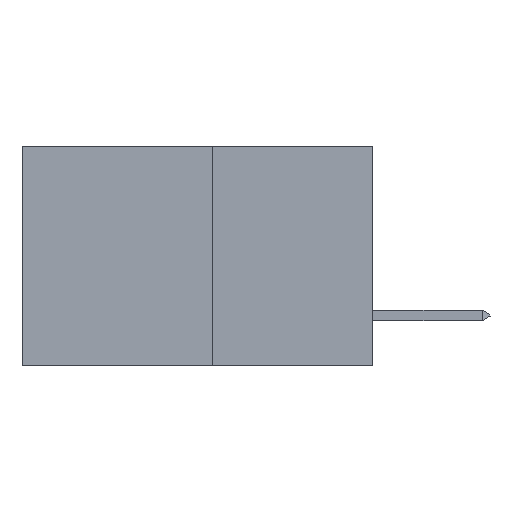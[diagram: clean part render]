
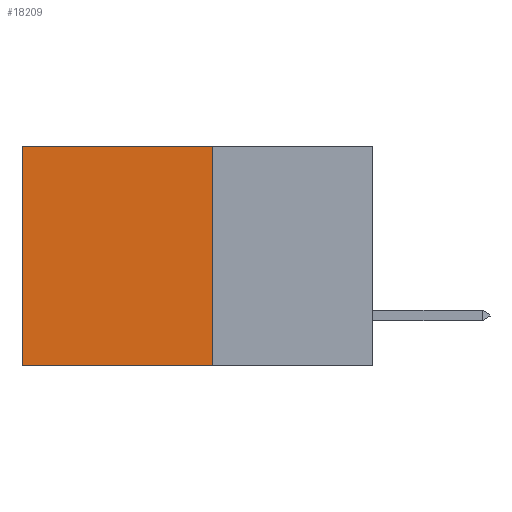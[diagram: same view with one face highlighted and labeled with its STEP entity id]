
A CAD part, left-side view. The second image highlights one B-rep face of the part: STEP entity #18209.
In plain terms, the highlighted planar face has unit normal (-1, 0, 0).
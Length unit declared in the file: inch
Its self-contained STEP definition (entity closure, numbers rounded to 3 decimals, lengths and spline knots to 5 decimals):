
#108 = EDGE_CURVE ( 'NONE', #5743, #16126, #417, .T. ) ;
#314 = DIRECTION ( 'NONE',  ( 0., 1., 0. ) ) ;
#417 = LINE ( 'NONE', #13929, #11786 ) ;
#859 = EDGE_CURVE ( 'NONE', #16126, #6185, #3263, .T. ) ;
#3263 = LINE ( 'NONE', #13642, #17883 ) ;
#4780 = EDGE_CURVE ( 'NONE', #5743, #17877, #18386, .T. ) ;
#4881 = DIRECTION ( 'NONE',  ( 0., 0., -1. ) ) ;
#4972 = EDGE_CURVE ( 'NONE', #17877, #6185, #6534, .T. ) ;
#5230 = CARTESIAN_POINT ( 'NONE',  ( 0.277, 0.27, -0.37 ) ) ;
#5395 = ORIENTED_EDGE ( 'NONE', *, *, #4780, .F. ) ;
#5743 = VERTEX_POINT ( 'NONE', #8380 ) ;
#6185 = VERTEX_POINT ( 'NONE', #18871 ) ;
#6534 = LINE ( 'NONE', #18498, #17705 ) ;
#7041 = DIRECTION ( 'NONE',  ( 0., 0., -1. ) ) ;
#7309 = ORIENTED_EDGE ( 'NONE', *, *, #108, .T. ) ;
#8380 = CARTESIAN_POINT ( 'NONE',  ( 0.277, 0.27, 0. ) ) ;
#9142 = AXIS2_PLACEMENT_3D ( 'NONE', #11398, #15782, #7041 ) ;
#9275 = EDGE_LOOP ( 'NONE', ( #14963, #17220, #5395, #7309 ) ) ;
#11398 = CARTESIAN_POINT ( 'NONE',  ( 0.277, 0.27, -0.37 ) ) ;
#11786 = VECTOR ( 'NONE', #15938, 39.37008 ) ;
#12770 = DIRECTION ( 'NONE',  ( 0., 0., -1. ) ) ;
#13642 = CARTESIAN_POINT ( 'NONE',  ( 0.277, 0.59, -0.37 ) ) ;
#13929 = CARTESIAN_POINT ( 'NONE',  ( 0.277, 0.27, 0. ) ) ;
#14116 = VECTOR ( 'NONE', #4881, 39.37008 ) ;
#14714 = CARTESIAN_POINT ( 'NONE',  ( 0.277, 0.59, 0. ) ) ;
#14963 = ORIENTED_EDGE ( 'NONE', *, *, #859, .T. ) ;
#15782 = DIRECTION ( 'NONE',  ( 1., 0., 0. ) ) ;
#15938 = DIRECTION ( 'NONE',  ( 0., 1., 0. ) ) ;
#16126 = VERTEX_POINT ( 'NONE', #14714 ) ;
#16228 = FACE_OUTER_BOUND ( 'NONE', #9275, .T. ) ;
#17220 = ORIENTED_EDGE ( 'NONE', *, *, #4972, .F. ) ;
#17705 = VECTOR ( 'NONE', #314, 39.37008 ) ;
#17877 = VERTEX_POINT ( 'NONE', #18555 ) ;
#17883 = VECTOR ( 'NONE', #12770, 39.37008 ) ;
#18209 = ADVANCED_FACE ( 'NONE', ( #16228 ), #18596, .F. ) ;
#18386 = LINE ( 'NONE', #5230, #14116 ) ;
#18498 = CARTESIAN_POINT ( 'NONE',  ( 0.277, 0.27, -0.37 ) ) ;
#18555 = CARTESIAN_POINT ( 'NONE',  ( 0.277, 0.27, -0.37 ) ) ;
#18596 = PLANE ( 'NONE',  #9142 ) ;
#18871 = CARTESIAN_POINT ( 'NONE',  ( 0.277, 0.59, -0.37 ) ) ;
